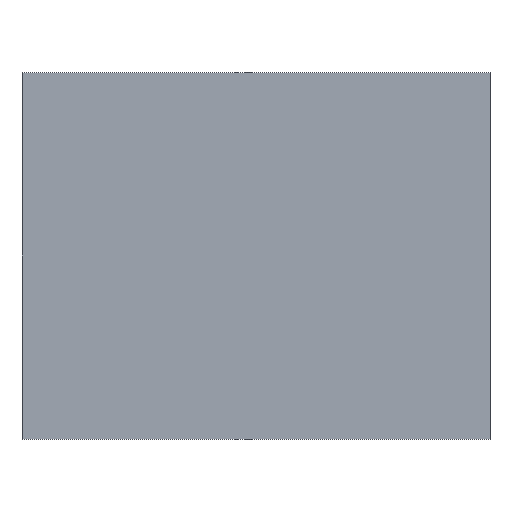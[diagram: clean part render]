
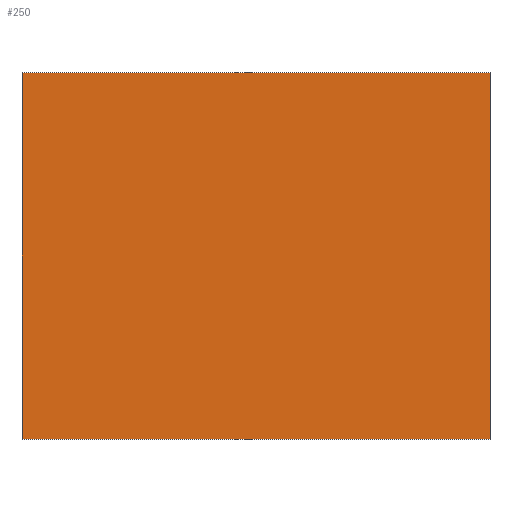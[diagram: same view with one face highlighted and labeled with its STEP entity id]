
A CAD part, left-side view. The second image highlights one B-rep face of the part: STEP entity #250.
In plain terms, the highlighted planar face has unit normal (-1, 0, 0).
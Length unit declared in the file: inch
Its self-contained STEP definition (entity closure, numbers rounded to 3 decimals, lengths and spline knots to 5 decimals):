
#19 = EDGE_LOOP ( 'NONE', ( #159, #285, #59, #26 ) ) ;
#21 = CARTESIAN_POINT ( 'NONE',  ( -0.22, 0., -0.54 ) ) ;
#26 = ORIENTED_EDGE ( 'NONE', *, *, #28, .T. ) ;
#28 = EDGE_CURVE ( 'NONE', #191, #245, #84, .T. ) ;
#47 = DIRECTION ( 'NONE',  ( 0., -1., 0. ) ) ;
#55 = CARTESIAN_POINT ( 'NONE',  ( -0.22, 0., 0.6 ) ) ;
#59 = ORIENTED_EDGE ( 'NONE', *, *, #71, .T. ) ;
#71 = EDGE_CURVE ( 'NONE', #212, #191, #317, .T. ) ;
#74 = VECTOR ( 'NONE', #47, 39.37008 ) ;
#80 = LINE ( 'NONE', #164, #74 ) ;
#82 = DIRECTION ( 'NONE',  ( -1., 0., 0. ) ) ;
#84 = LINE ( 'NONE', #88, #178 ) ;
#88 = CARTESIAN_POINT ( 'NONE',  ( -0.22, 1.45472, -0.54 ) ) ;
#102 = DIRECTION ( 'NONE',  ( 0., 0., 1. ) ) ;
#128 = PLANE ( 'NONE',  #315 ) ;
#131 = EDGE_CURVE ( 'NONE', #212, #328, #80, .T. ) ;
#144 = CARTESIAN_POINT ( 'NONE',  ( -0.22, 0., 0. ) ) ;
#145 = DIRECTION ( 'NONE',  ( 0., 0., -1. ) ) ;
#159 = ORIENTED_EDGE ( 'NONE', *, *, #222, .F. ) ;
#164 = CARTESIAN_POINT ( 'NONE',  ( -0.22, 1.45472, 0.6 ) ) ;
#178 = VECTOR ( 'NONE', #263, 39.37008 ) ;
#191 = VERTEX_POINT ( 'NONE', #271 ) ;
#193 = CARTESIAN_POINT ( 'NONE',  ( -0.22, 1.45472, 0.6 ) ) ;
#210 = VECTOR ( 'NONE', #145, 39.37008 ) ;
#212 = VERTEX_POINT ( 'NONE', #193 ) ;
#222 = EDGE_CURVE ( 'NONE', #328, #245, #231, .T. ) ;
#223 = CARTESIAN_POINT ( 'NONE',  ( -0.22, 1.45472, 0. ) ) ;
#231 = LINE ( 'NONE', #144, #210 ) ;
#245 = VERTEX_POINT ( 'NONE', #21 ) ;
#250 = ADVANCED_FACE ( 'NONE', ( #301 ), #128, .T. ) ;
#263 = DIRECTION ( 'NONE',  ( 0., -1., 0. ) ) ;
#267 = CARTESIAN_POINT ( 'NONE',  ( -0.22, 1.45472, 0. ) ) ;
#271 = CARTESIAN_POINT ( 'NONE',  ( -0.22, 1.45472, -0.54 ) ) ;
#285 = ORIENTED_EDGE ( 'NONE', *, *, #131, .F. ) ;
#301 = FACE_OUTER_BOUND ( 'NONE', #19, .T. ) ;
#309 = VECTOR ( 'NONE', #320, 39.37008 ) ;
#315 = AXIS2_PLACEMENT_3D ( 'NONE', #223, #82, #102 ) ;
#317 = LINE ( 'NONE', #267, #309 ) ;
#320 = DIRECTION ( 'NONE',  ( 0., 0., -1. ) ) ;
#328 = VERTEX_POINT ( 'NONE', #55 ) ;
